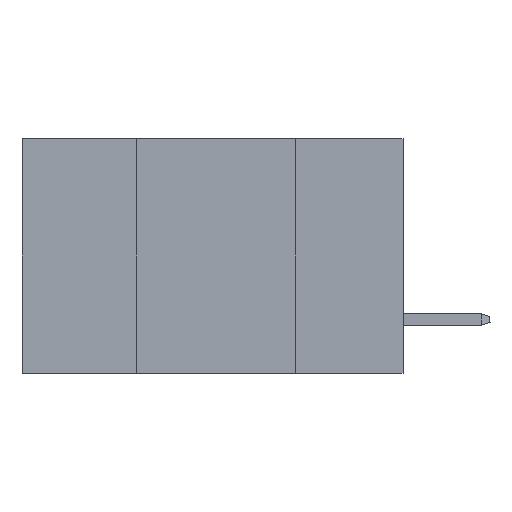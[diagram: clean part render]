
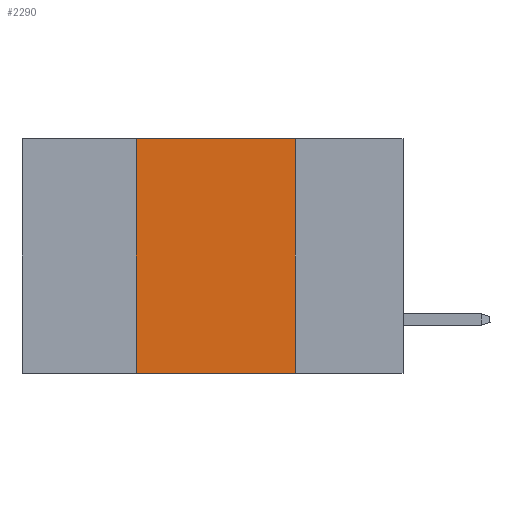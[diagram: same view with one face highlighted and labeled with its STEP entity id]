
A CAD part, left-side view. The second image highlights one B-rep face of the part: STEP entity #2290.
In plain terms, the highlighted planar face has unit normal (-1, 0, 0).
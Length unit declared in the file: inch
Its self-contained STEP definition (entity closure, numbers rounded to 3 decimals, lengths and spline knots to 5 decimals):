
#477 = DIRECTION ( 'NONE',  ( 0., 0., -1. ) ) ;
#956 = VECTOR ( 'NONE', #32628, 39.37008 ) ;
#1403 = EDGE_CURVE ( 'NONE', #21228, #33855, #6416, .T. ) ;
#2290 = ADVANCED_FACE ( 'NONE', ( #24059 ), #36362, .F. ) ;
#3314 = EDGE_CURVE ( 'NONE', #33855, #3392, #31350, .T. ) ;
#3392 = VERTEX_POINT ( 'NONE', #19201 ) ;
#4237 = CARTESIAN_POINT ( 'NONE',  ( 0., 0.6, -0.37 ) ) ;
#4272 = VECTOR ( 'NONE', #22790, 39.37008 ) ;
#5288 = DIRECTION ( 'NONE',  ( 0., 0., -1. ) ) ;
#6132 = VERTEX_POINT ( 'NONE', #26278 ) ;
#6329 = CARTESIAN_POINT ( 'NONE',  ( 0., 0.17, 0. ) ) ;
#6416 = LINE ( 'NONE', #7597, #956 ) ;
#6835 = AXIS2_PLACEMENT_3D ( 'NONE', #20602, #14747, #5288 ) ;
#7597 = CARTESIAN_POINT ( 'NONE',  ( 0., 0.6, 0. ) ) ;
#8735 = CARTESIAN_POINT ( 'NONE',  ( 0., 0.42, 0. ) ) ;
#14747 = DIRECTION ( 'NONE',  ( 1., 0., 0. ) ) ;
#14837 = VECTOR ( 'NONE', #477, 39.37008 ) ;
#15594 = ORIENTED_EDGE ( 'NONE', *, *, #1403, .F. ) ;
#16773 = LINE ( 'NONE', #29106, #35198 ) ;
#18395 = ORIENTED_EDGE ( 'NONE', *, *, #30697, .F. ) ;
#19201 = CARTESIAN_POINT ( 'NONE',  ( 0., 0.17, -0.37 ) ) ;
#19359 = LINE ( 'NONE', #4237, #4272 ) ;
#20602 = CARTESIAN_POINT ( 'NONE',  ( 0., 0.6, 0. ) ) ;
#21228 = VERTEX_POINT ( 'NONE', #8735 ) ;
#21236 = CARTESIAN_POINT ( 'NONE',  ( 0., 0.17, 0. ) ) ;
#22790 = DIRECTION ( 'NONE',  ( 0., -1., 0. ) ) ;
#24059 = FACE_OUTER_BOUND ( 'NONE', #26940, .T. ) ;
#26278 = CARTESIAN_POINT ( 'NONE',  ( 0., 0.42, -0.37 ) ) ;
#26940 = EDGE_LOOP ( 'NONE', ( #29525, #15594, #18395, #39365 ) ) ;
#29106 = CARTESIAN_POINT ( 'NONE',  ( 0., 0.42, 0. ) ) ;
#29511 = DIRECTION ( 'NONE',  ( 0., 0., 1. ) ) ;
#29525 = ORIENTED_EDGE ( 'NONE', *, *, #3314, .F. ) ;
#30697 = EDGE_CURVE ( 'NONE', #6132, #21228, #16773, .T. ) ;
#30990 = EDGE_CURVE ( 'NONE', #6132, #3392, #19359, .T. ) ;
#31350 = LINE ( 'NONE', #6329, #14837 ) ;
#32628 = DIRECTION ( 'NONE',  ( 0., -1., 0. ) ) ;
#33855 = VERTEX_POINT ( 'NONE', #21236 ) ;
#35198 = VECTOR ( 'NONE', #29511, 39.37008 ) ;
#36362 = PLANE ( 'NONE',  #6835 ) ;
#39365 = ORIENTED_EDGE ( 'NONE', *, *, #30990, .T. ) ;
